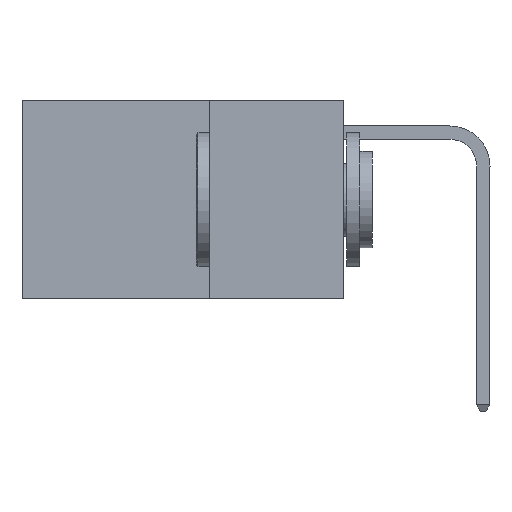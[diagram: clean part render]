
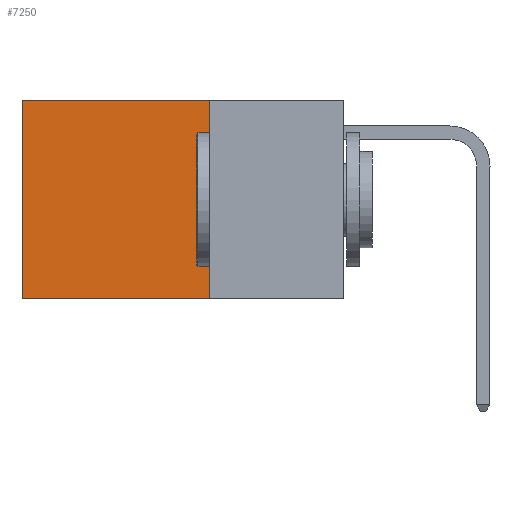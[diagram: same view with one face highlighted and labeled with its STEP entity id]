
A CAD part, left-side view. The second image highlights one B-rep face of the part: STEP entity #7250.
In plain terms, the highlighted planar face has unit normal (-1, 0, 0).
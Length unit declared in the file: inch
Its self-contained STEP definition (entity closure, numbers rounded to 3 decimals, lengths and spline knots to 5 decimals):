
#103 = CARTESIAN_POINT ( 'NONE',  ( 0.2625, 0.25, -0.37 ) ) ;
#310 = EDGE_CURVE ( 'NONE', #9368, #862, #5887, .T. ) ;
#331 = VECTOR ( 'NONE', #11130, 39.37008 ) ;
#648 = VECTOR ( 'NONE', #8363, 39.37008 ) ;
#862 = VERTEX_POINT ( 'NONE', #103 ) ;
#1687 = AXIS2_PLACEMENT_3D ( 'NONE', #9839, #1688, #8118 ) ;
#1688 = DIRECTION ( 'NONE',  ( 1., 0., 0. ) ) ;
#2823 = VECTOR ( 'NONE', #6087, 39.37008 ) ;
#2854 = CARTESIAN_POINT ( 'NONE',  ( 0.2625, 0.25, 0. ) ) ;
#3677 = CARTESIAN_POINT ( 'NONE',  ( 0.2625, 0.6, 0. ) ) ;
#5075 = ORIENTED_EDGE ( 'NONE', *, *, #10732, .T. ) ;
#5152 = CARTESIAN_POINT ( 'NONE',  ( 0.2625, 0.25, -0.37 ) ) ;
#5265 = LINE ( 'NONE', #5152, #2823 ) ;
#5785 = CARTESIAN_POINT ( 'NONE',  ( 0.2625, 0.6, -0.37 ) ) ;
#5840 = EDGE_LOOP ( 'NONE', ( #5075, #6008, #6084, #6174 ) ) ;
#5887 = LINE ( 'NONE', #7757, #331 ) ;
#6008 = ORIENTED_EDGE ( 'NONE', *, *, #11162, .F. ) ;
#6084 = ORIENTED_EDGE ( 'NONE', *, *, #310, .F. ) ;
#6087 = DIRECTION ( 'NONE',  ( 0., 1., 0. ) ) ;
#6174 = ORIENTED_EDGE ( 'NONE', *, *, #8079, .T. ) ;
#6970 = VECTOR ( 'NONE', #9981, 39.37008 ) ;
#7250 = ADVANCED_FACE ( 'NONE', ( #9827 ), #10692, .F. ) ;
#7757 = CARTESIAN_POINT ( 'NONE',  ( 0.2625, 0.25, 0. ) ) ;
#8017 = LINE ( 'NONE', #2854, #648 ) ;
#8079 = EDGE_CURVE ( 'NONE', #9368, #9531, #8017, .T. ) ;
#8118 = DIRECTION ( 'NONE',  ( 0., 0., -1. ) ) ;
#8256 = CARTESIAN_POINT ( 'NONE',  ( 0.2625, 0.6, 0. ) ) ;
#8363 = DIRECTION ( 'NONE',  ( 0., 1., 0. ) ) ;
#8726 = VERTEX_POINT ( 'NONE', #5785 ) ;
#8782 = LINE ( 'NONE', #3677, #6970 ) ;
#9368 = VERTEX_POINT ( 'NONE', #10639 ) ;
#9531 = VERTEX_POINT ( 'NONE', #8256 ) ;
#9827 = FACE_OUTER_BOUND ( 'NONE', #5840, .T. ) ;
#9839 = CARTESIAN_POINT ( 'NONE',  ( 0.2625, 0.25, 0. ) ) ;
#9981 = DIRECTION ( 'NONE',  ( 0., 0., -1. ) ) ;
#10639 = CARTESIAN_POINT ( 'NONE',  ( 0.2625, 0.25, 0. ) ) ;
#10692 = PLANE ( 'NONE',  #1687 ) ;
#10732 = EDGE_CURVE ( 'NONE', #9531, #8726, #8782, .T. ) ;
#11130 = DIRECTION ( 'NONE',  ( 0., 0., -1. ) ) ;
#11162 = EDGE_CURVE ( 'NONE', #862, #8726, #5265, .T. ) ;
